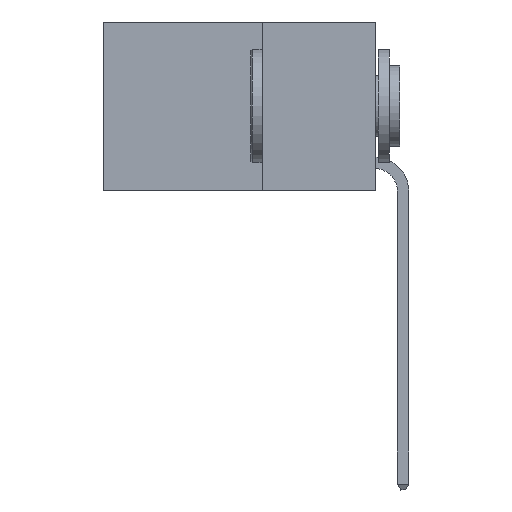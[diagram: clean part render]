
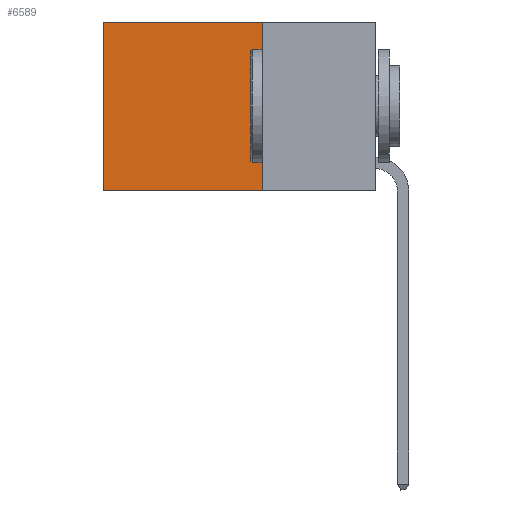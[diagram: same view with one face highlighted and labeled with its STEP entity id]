
A CAD part, left-side view. The second image highlights one B-rep face of the part: STEP entity #6589.
In plain terms, the highlighted planar face has unit normal (-1, 0, 0).
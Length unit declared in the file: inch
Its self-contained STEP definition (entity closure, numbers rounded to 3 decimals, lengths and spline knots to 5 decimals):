
#865 = ORIENTED_EDGE ( 'NONE', *, *, #21589, .T. ) ;
#1191 = CARTESIAN_POINT ( 'NONE',  ( 0.2625, 0.25, 0. ) ) ;
#1337 = DIRECTION ( 'NONE',  ( 0., 0., -1. ) ) ;
#2398 = CARTESIAN_POINT ( 'NONE',  ( 0.2625, 0.25, -0.37 ) ) ;
#2643 = VECTOR ( 'NONE', #1337, 39.37008 ) ;
#4758 = VERTEX_POINT ( 'NONE', #6631 ) ;
#4827 = DIRECTION ( 'NONE',  ( 1., 0., 0. ) ) ;
#5466 = LINE ( 'NONE', #8903, #18693 ) ;
#6168 = EDGE_CURVE ( 'NONE', #8608, #16154, #16679, .T. ) ;
#6513 = CARTESIAN_POINT ( 'NONE',  ( 0.2625, 0.25, -0.37 ) ) ;
#6589 = ADVANCED_FACE ( 'NONE', ( #8051 ), #19789, .F. ) ;
#6631 = CARTESIAN_POINT ( 'NONE',  ( 0.2625, 0.6, 0. ) ) ;
#7243 = DIRECTION ( 'NONE',  ( 0., 0., -1. ) ) ;
#7743 = ORIENTED_EDGE ( 'NONE', *, *, #15935, .F. ) ;
#7823 = VECTOR ( 'NONE', #13370, 39.37008 ) ;
#8051 = FACE_OUTER_BOUND ( 'NONE', #17064, .T. ) ;
#8284 = LINE ( 'NONE', #15019, #2643 ) ;
#8608 = VERTEX_POINT ( 'NONE', #2398 ) ;
#8903 = CARTESIAN_POINT ( 'NONE',  ( 0.2625, 0.6, 0. ) ) ;
#9677 = DIRECTION ( 'NONE',  ( 0., 0., -1. ) ) ;
#12742 = DIRECTION ( 'NONE',  ( 0., 1., 0. ) ) ;
#13370 = DIRECTION ( 'NONE',  ( 0., 1., 0. ) ) ;
#13675 = CARTESIAN_POINT ( 'NONE',  ( 0.2625, 0.25, 0. ) ) ;
#14824 = LINE ( 'NONE', #21623, #17273 ) ;
#15019 = CARTESIAN_POINT ( 'NONE',  ( 0.2625, 0.25, 0. ) ) ;
#15590 = ORIENTED_EDGE ( 'NONE', *, *, #6168, .F. ) ;
#15846 = AXIS2_PLACEMENT_3D ( 'NONE', #1191, #4827, #9677 ) ;
#15935 = EDGE_CURVE ( 'NONE', #17602, #8608, #8284, .T. ) ;
#15995 = ORIENTED_EDGE ( 'NONE', *, *, #21339, .T. ) ;
#16154 = VERTEX_POINT ( 'NONE', #21217 ) ;
#16679 = LINE ( 'NONE', #6513, #7823 ) ;
#17064 = EDGE_LOOP ( 'NONE', ( #15995, #15590, #7743, #865 ) ) ;
#17273 = VECTOR ( 'NONE', #12742, 39.37008 ) ;
#17602 = VERTEX_POINT ( 'NONE', #13675 ) ;
#18693 = VECTOR ( 'NONE', #7243, 39.37008 ) ;
#19789 = PLANE ( 'NONE',  #15846 ) ;
#21217 = CARTESIAN_POINT ( 'NONE',  ( 0.2625, 0.6, -0.37 ) ) ;
#21339 = EDGE_CURVE ( 'NONE', #4758, #16154, #5466, .T. ) ;
#21589 = EDGE_CURVE ( 'NONE', #17602, #4758, #14824, .T. ) ;
#21623 = CARTESIAN_POINT ( 'NONE',  ( 0.2625, 0.25, 0. ) ) ;
